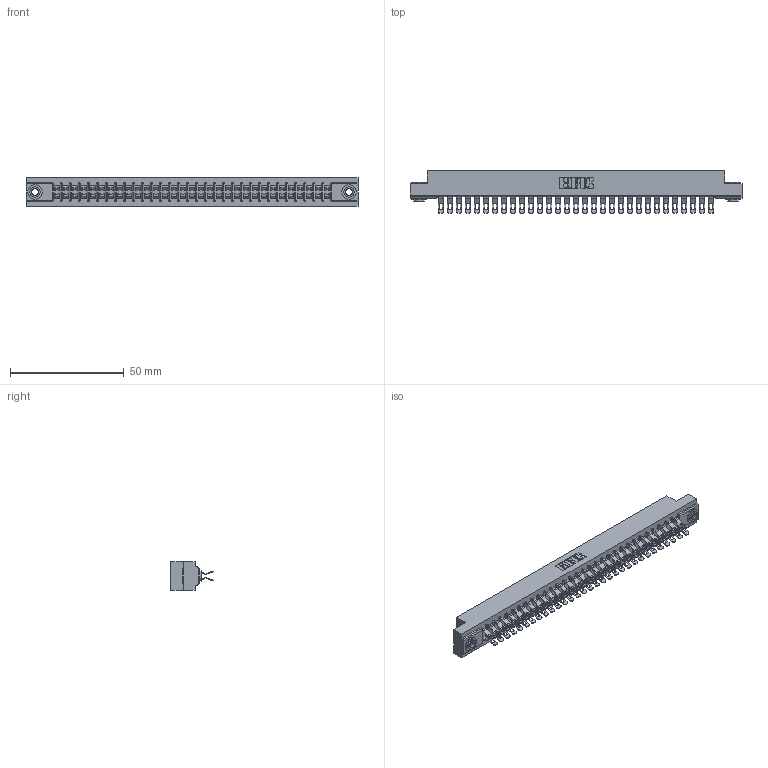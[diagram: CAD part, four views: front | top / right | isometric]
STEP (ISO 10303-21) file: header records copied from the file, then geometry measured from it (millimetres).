
FILE_DESCRIPTION (( 'STEP AP203' ), '1' );
FILE_NAME ('357-062-555-203.STEP', '2019-09-19T07:03:14', ( '' ), ( '' ), 'SwSTEP 2.0', 'SolidWorks 2016', '' );
FILE_SCHEMA (( 'CONFIG_CONTROL_DESIGN' ));
Length unit declared in the file: inch
Products named in the file (4): 307 Part_.156 Dia Mounting Holes; 345-250-002_345-250-002-102; 357-062-555-203; 307-290-001_555
Assembly tree (65 placements, depth 2):
  357-062-555-203
    307 Part_.156 Dia Mounting Holes
    307-290-001_555  x62
    345-250-002_345-250-002-102  x2
Bounding box: 145.85 x 18.75 x 12.7 mm (x, y, z)
Volume: 15617.2 mm3; surface area: 20162.2 mm2
Topology: 65 solids, 65 shells, 3984 faces, 11657 edges, 7598 vertices
Faces by surface type: plane 2202, cylinder 1710, sphere 64, cone 8
Entity records: 30526 total; most frequent: CARTESIAN_POINT 4984, ORIENTED_EDGE 4932, DIRECTION 4908, EDGE_CURVE 2466, LINE 1868, VECTOR 1868, VERTEX_POINT 1596, AXIS2_PLACEMENT_3D 1520
